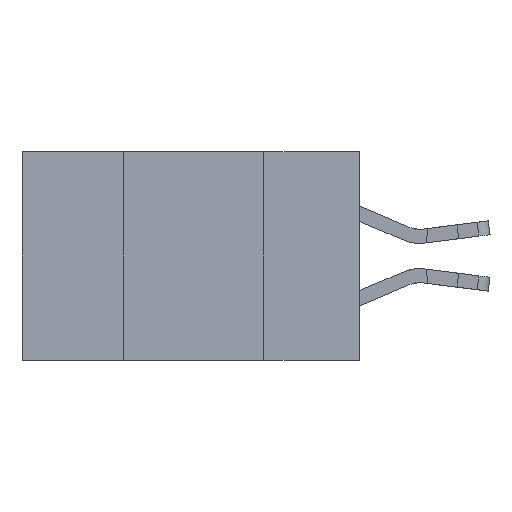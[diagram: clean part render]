
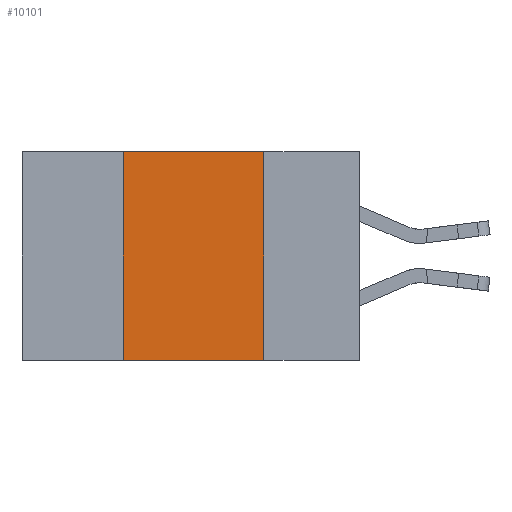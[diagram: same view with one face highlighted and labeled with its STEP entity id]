
A CAD part, left-side view. The second image highlights one B-rep face of the part: STEP entity #10101.
In plain terms, the highlighted planar face has unit normal (-1, 0, 0).
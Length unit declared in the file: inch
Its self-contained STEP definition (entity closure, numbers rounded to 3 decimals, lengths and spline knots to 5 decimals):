
#534 = CARTESIAN_POINT ( 'NONE',  ( 0., 0.6, 0. ) ) ;
#1128 = CARTESIAN_POINT ( 'NONE',  ( 0., 0.42, 0. ) ) ;
#1712 = EDGE_CURVE ( 'NONE', #9322, #5847, #12237, .T. ) ;
#2373 = CARTESIAN_POINT ( 'NONE',  ( 0., 0.42, -0.37 ) ) ;
#2474 = VECTOR ( 'NONE', #6136, 39.37008 ) ;
#2491 = VERTEX_POINT ( 'NONE', #7614 ) ;
#2662 = VECTOR ( 'NONE', #9954, 39.37008 ) ;
#2833 = DIRECTION ( 'NONE',  ( 0., 0., -1. ) ) ;
#3060 = LINE ( 'NONE', #1128, #2662 ) ;
#3556 = CARTESIAN_POINT ( 'NONE',  ( 0., 0.17, -0.37 ) ) ;
#4447 = PLANE ( 'NONE',  #4944 ) ;
#4689 = VECTOR ( 'NONE', #11957, 39.37008 ) ;
#4944 = AXIS2_PLACEMENT_3D ( 'NONE', #534, #12888, #5736 ) ;
#5736 = DIRECTION ( 'NONE',  ( 0., 0., -1. ) ) ;
#5847 = VERTEX_POINT ( 'NONE', #3556 ) ;
#5875 = FACE_OUTER_BOUND ( 'NONE', #6917, .T. ) ;
#6136 = DIRECTION ( 'NONE',  ( 0., -1., 0. ) ) ;
#6917 = EDGE_LOOP ( 'NONE', ( #14319, #9245, #12298, #7529 ) ) ;
#7529 = ORIENTED_EDGE ( 'NONE', *, *, #14261, .T. ) ;
#7614 = CARTESIAN_POINT ( 'NONE',  ( 0., 0.42, 0. ) ) ;
#7655 = LINE ( 'NONE', #8505, #4689 ) ;
#8505 = CARTESIAN_POINT ( 'NONE',  ( 0., 0.6, -0.37 ) ) ;
#9169 = VECTOR ( 'NONE', #2833, 39.37008 ) ;
#9180 = LINE ( 'NONE', #14440, #2474 ) ;
#9245 = ORIENTED_EDGE ( 'NONE', *, *, #9683, .F. ) ;
#9322 = VERTEX_POINT ( 'NONE', #14803 ) ;
#9683 = EDGE_CURVE ( 'NONE', #2491, #9322, #9180, .T. ) ;
#9724 = VERTEX_POINT ( 'NONE', #2373 ) ;
#9954 = DIRECTION ( 'NONE',  ( 0., 0., 1. ) ) ;
#10101 = ADVANCED_FACE ( 'NONE', ( #5875 ), #4447, .F. ) ;
#11957 = DIRECTION ( 'NONE',  ( 0., -1., 0. ) ) ;
#12237 = LINE ( 'NONE', #12948, #9169 ) ;
#12298 = ORIENTED_EDGE ( 'NONE', *, *, #14361, .F. ) ;
#12888 = DIRECTION ( 'NONE',  ( 1., 0., 0. ) ) ;
#12948 = CARTESIAN_POINT ( 'NONE',  ( 0., 0.17, 0. ) ) ;
#14261 = EDGE_CURVE ( 'NONE', #9724, #5847, #7655, .T. ) ;
#14319 = ORIENTED_EDGE ( 'NONE', *, *, #1712, .F. ) ;
#14361 = EDGE_CURVE ( 'NONE', #9724, #2491, #3060, .T. ) ;
#14440 = CARTESIAN_POINT ( 'NONE',  ( 0., 0.6, 0. ) ) ;
#14803 = CARTESIAN_POINT ( 'NONE',  ( 0., 0.17, 0. ) ) ;
